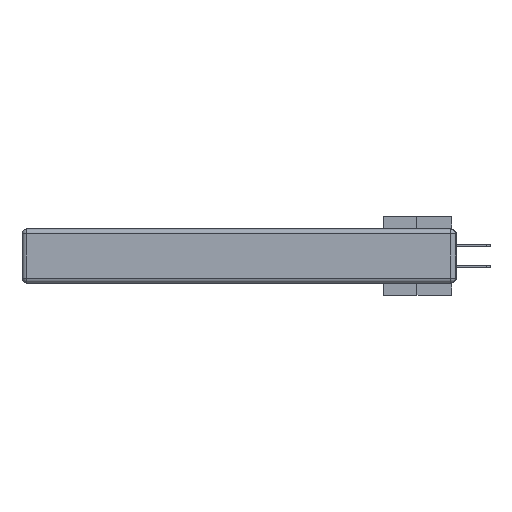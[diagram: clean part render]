
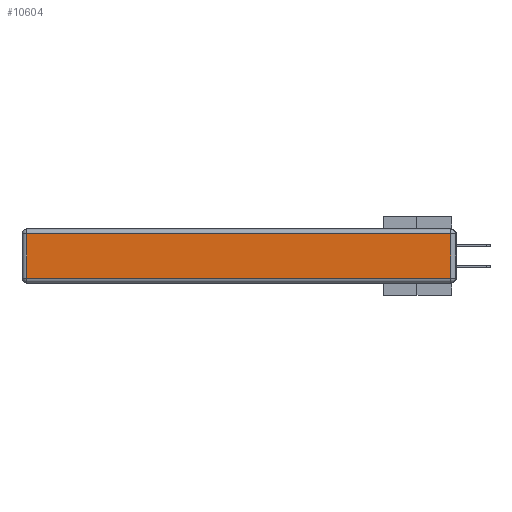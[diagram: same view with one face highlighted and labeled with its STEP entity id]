
A CAD part, left-side view. The second image highlights one B-rep face of the part: STEP entity #10604.
In plain terms, the highlighted planar face has unit normal (-1, 0, 0).
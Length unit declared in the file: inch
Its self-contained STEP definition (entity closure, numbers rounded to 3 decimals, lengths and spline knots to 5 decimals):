
#513 = VECTOR ( 'NONE', #25940, 39.37008 ) ;
#3614 = CARTESIAN_POINT ( 'NONE',  ( 0., 2.72, -0.313 ) ) ;
#6818 = CARTESIAN_POINT ( 'NONE',  ( 0., 0., -0.343 ) ) ;
#7340 = ORIENTED_EDGE ( 'NONE', *, *, #18964, .T. ) ;
#9910 = AXIS2_PLACEMENT_3D ( 'NONE', #6818, #23086, #12442 ) ;
#10604 = ADVANCED_FACE ( 'NONE', ( #14952 ), #14774, .T. ) ;
#12091 = LINE ( 'NONE', #23505, #34220 ) ;
#12442 = DIRECTION ( 'NONE',  ( 0., 0., 1. ) ) ;
#13752 = LINE ( 'NONE', #14257, #32565 ) ;
#14257 = CARTESIAN_POINT ( 'NONE',  ( 0., 0.03, -0.343 ) ) ;
#14774 = PLANE ( 'NONE',  #9910 ) ;
#14952 = FACE_OUTER_BOUND ( 'NONE', #26689, .T. ) ;
#15247 = VERTEX_POINT ( 'NONE', #22912 ) ;
#15310 = DIRECTION ( 'NONE',  ( 0., 1., 0. ) ) ;
#15791 = ORIENTED_EDGE ( 'NONE', *, *, #22621, .T. ) ;
#17390 = LINE ( 'NONE', #28703, #27427 ) ;
#17825 = ORIENTED_EDGE ( 'NONE', *, *, #18020, .T. ) ;
#18020 = EDGE_CURVE ( 'NONE', #33400, #28340, #17390, .T. ) ;
#18964 = EDGE_CURVE ( 'NONE', #15247, #33400, #28211, .T. ) ;
#20163 = VERTEX_POINT ( 'NONE', #22364 ) ;
#21024 = DIRECTION ( 'NONE',  ( 0., -1., 0. ) ) ;
#22364 = CARTESIAN_POINT ( 'NONE',  ( 0., 0.03, -0.03 ) ) ;
#22621 = EDGE_CURVE ( 'NONE', #28340, #20163, #13752, .T. ) ;
#22912 = CARTESIAN_POINT ( 'NONE',  ( 0., 2.72, -0.03 ) ) ;
#23086 = DIRECTION ( 'NONE',  ( -1., 0., 0. ) ) ;
#23505 = CARTESIAN_POINT ( 'NONE',  ( 0., 2.75, -0.03 ) ) ;
#25827 = CARTESIAN_POINT ( 'NONE',  ( 0., 2.72, -0.343 ) ) ;
#25940 = DIRECTION ( 'NONE',  ( 0., 0., -1. ) ) ;
#26689 = EDGE_LOOP ( 'NONE', ( #17825, #15791, #34288, #7340 ) ) ;
#27427 = VECTOR ( 'NONE', #21024, 39.37008 ) ;
#28211 = LINE ( 'NONE', #25827, #513 ) ;
#28227 = CARTESIAN_POINT ( 'NONE',  ( 0., 0.03, -0.313 ) ) ;
#28340 = VERTEX_POINT ( 'NONE', #28227 ) ;
#28703 = CARTESIAN_POINT ( 'NONE',  ( 0., 0., -0.313 ) ) ;
#29863 = EDGE_CURVE ( 'NONE', #20163, #15247, #12091, .T. ) ;
#32565 = VECTOR ( 'NONE', #33062, 39.37008 ) ;
#33062 = DIRECTION ( 'NONE',  ( 0., 0., 1. ) ) ;
#33400 = VERTEX_POINT ( 'NONE', #3614 ) ;
#34220 = VECTOR ( 'NONE', #15310, 39.37008 ) ;
#34288 = ORIENTED_EDGE ( 'NONE', *, *, #29863, .T. ) ;
